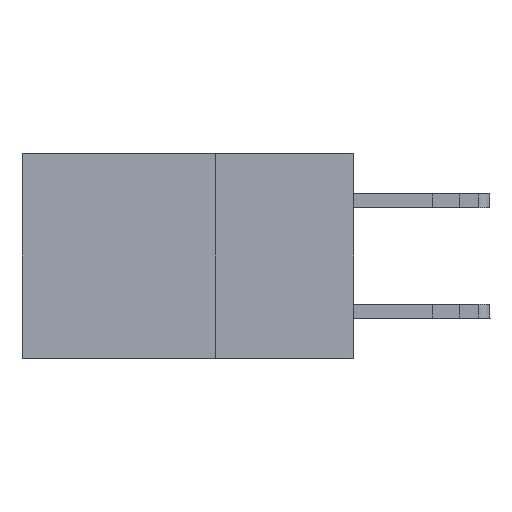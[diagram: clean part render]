
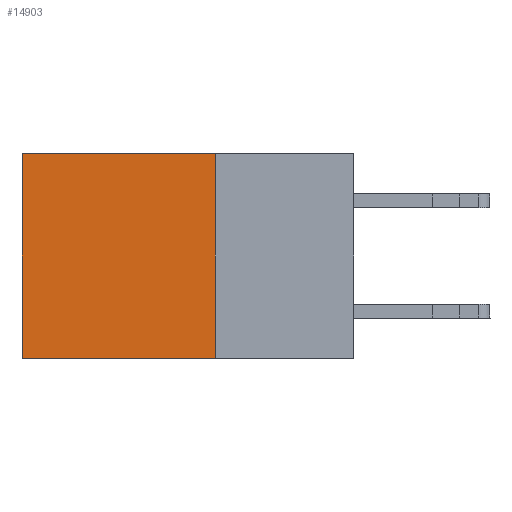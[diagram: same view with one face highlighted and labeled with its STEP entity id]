
A CAD part, left-side view. The second image highlights one B-rep face of the part: STEP entity #14903.
In plain terms, the highlighted planar face has unit normal (-1, 0, 0).
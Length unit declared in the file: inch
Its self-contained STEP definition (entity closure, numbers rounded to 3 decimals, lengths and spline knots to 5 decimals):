
#230 = ORIENTED_EDGE ( 'NONE', *, *, #12421, .F. ) ;
#863 = CARTESIAN_POINT ( 'NONE',  ( 0.2875, 0.6, 0. ) ) ;
#1136 = DIRECTION ( 'NONE',  ( 0., 0., -1. ) ) ;
#2317 = FACE_OUTER_BOUND ( 'NONE', #6293, .T. ) ;
#2664 = CARTESIAN_POINT ( 'NONE',  ( 0.2875, 0.6, -0.37 ) ) ;
#3535 = VERTEX_POINT ( 'NONE', #11024 ) ;
#3679 = CARTESIAN_POINT ( 'NONE',  ( 0.2875, 0.25, 0. ) ) ;
#3981 = CARTESIAN_POINT ( 'NONE',  ( 0.2875, 0.6, 0. ) ) ;
#4562 = DIRECTION ( 'NONE',  ( 0., 1., 0. ) ) ;
#4857 = VECTOR ( 'NONE', #6046, 39.37008 ) ;
#6046 = DIRECTION ( 'NONE',  ( 0., 1., 0. ) ) ;
#6293 = EDGE_LOOP ( 'NONE', ( #12140, #6898, #230, #7076 ) ) ;
#6898 = ORIENTED_EDGE ( 'NONE', *, *, #14480, .F. ) ;
#7052 = CARTESIAN_POINT ( 'NONE',  ( 0.2875, 0.25, 0. ) ) ;
#7076 = ORIENTED_EDGE ( 'NONE', *, *, #14789, .T. ) ;
#7182 = DIRECTION ( 'NONE',  ( 0., 0., -1. ) ) ;
#7232 = CARTESIAN_POINT ( 'NONE',  ( 0.2875, 0.25, -0.37 ) ) ;
#7796 = LINE ( 'NONE', #863, #11045 ) ;
#7872 = VERTEX_POINT ( 'NONE', #3981 ) ;
#8202 = VERTEX_POINT ( 'NONE', #2664 ) ;
#9749 = VERTEX_POINT ( 'NONE', #7232 ) ;
#9773 = VECTOR ( 'NONE', #7182, 39.37008 ) ;
#10212 = DIRECTION ( 'NONE',  ( 0., 0., -1. ) ) ;
#11024 = CARTESIAN_POINT ( 'NONE',  ( 0.2875, 0.25, 0. ) ) ;
#11045 = VECTOR ( 'NONE', #10212, 39.37008 ) ;
#11801 = DIRECTION ( 'NONE',  ( 1., 0., 0. ) ) ;
#11881 = PLANE ( 'NONE',  #12837 ) ;
#12140 = ORIENTED_EDGE ( 'NONE', *, *, #14031, .T. ) ;
#12421 = EDGE_CURVE ( 'NONE', #3535, #9749, #13013, .T. ) ;
#12837 = AXIS2_PLACEMENT_3D ( 'NONE', #7052, #11801, #1136 ) ;
#13013 = LINE ( 'NONE', #3679, #9773 ) ;
#13133 = LINE ( 'NONE', #15229, #14813 ) ;
#14031 = EDGE_CURVE ( 'NONE', #7872, #8202, #7796, .T. ) ;
#14218 = LINE ( 'NONE', #15248, #4857 ) ;
#14480 = EDGE_CURVE ( 'NONE', #9749, #8202, #14218, .T. ) ;
#14789 = EDGE_CURVE ( 'NONE', #3535, #7872, #13133, .T. ) ;
#14813 = VECTOR ( 'NONE', #4562, 39.37008 ) ;
#14903 = ADVANCED_FACE ( 'NONE', ( #2317 ), #11881, .F. ) ;
#15229 = CARTESIAN_POINT ( 'NONE',  ( 0.2875, 0.25, 0. ) ) ;
#15248 = CARTESIAN_POINT ( 'NONE',  ( 0.2875, 0.25, -0.37 ) ) ;
